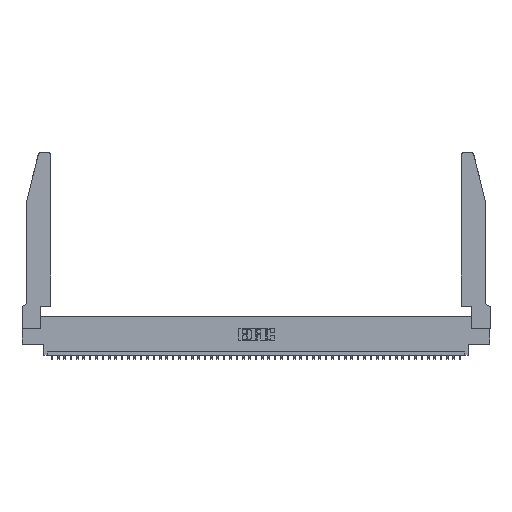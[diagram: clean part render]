
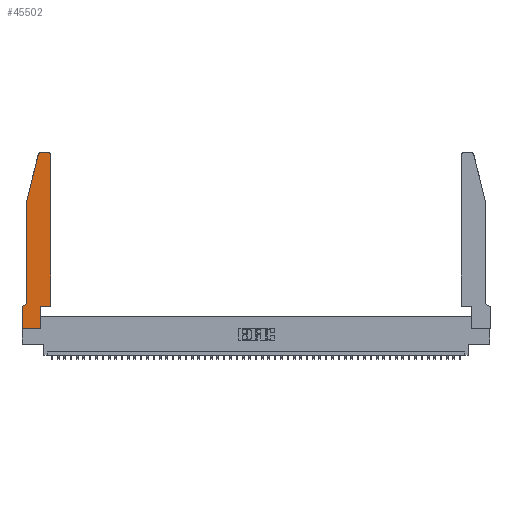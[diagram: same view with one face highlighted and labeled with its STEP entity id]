
A CAD part, top view. The second image highlights one B-rep face of the part: STEP entity #45502.
In plain terms, the highlighted planar face has unit normal (0, 0, 1).
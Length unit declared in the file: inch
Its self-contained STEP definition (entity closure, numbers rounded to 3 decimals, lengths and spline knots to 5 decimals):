
#623 = ORIENTED_EDGE ( 'NONE', *, *, #5632, .T. ) ;
#687 = VECTOR ( 'NONE', #29431, 39.37008 ) ;
#1785 = VECTOR ( 'NONE', #20263, 39.37008 ) ;
#2101 = CARTESIAN_POINT ( 'NONE',  ( 0.0755, 0.35, 0.37 ) ) ;
#2113 = VERTEX_POINT ( 'NONE', #43645 ) ;
#3459 = DIRECTION ( 'NONE',  ( 0., 1., 0. ) ) ;
#4169 = VERTEX_POINT ( 'NONE', #6044 ) ;
#4292 = EDGE_CURVE ( 'NONE', #4169, #29714, #37323, .T. ) ;
#4338 = ORIENTED_EDGE ( 'NONE', *, *, #27550, .T. ) ;
#5632 = EDGE_CURVE ( 'NONE', #13591, #13828, #32533, .T. ) ;
#5811 = VECTOR ( 'NONE', #3459, 39.37008 ) ;
#6044 = CARTESIAN_POINT ( 'NONE',  ( 0.2865, 0.35, 0.37 ) ) ;
#6108 = CARTESIAN_POINT ( 'NONE',  ( 0.4505, 2.72, 0.37 ) ) ;
#6437 = EDGE_CURVE ( 'NONE', #47533, #32549, #17622, .T. ) ;
#6633 = CARTESIAN_POINT ( 'NONE',  ( 0.4205, 2.75, 0.37 ) ) ;
#7588 = CARTESIAN_POINT ( 'NONE',  ( 0.284, 2.75, 0.37 ) ) ;
#7615 = ORIENTED_EDGE ( 'NONE', *, *, #19950, .T. ) ;
#7971 = CIRCLE ( 'NONE', #9192, 0.03 ) ;
#8495 = ORIENTED_EDGE ( 'NONE', *, *, #27144, .T. ) ;
#9192 = AXIS2_PLACEMENT_3D ( 'NONE', #14152, #41817, #18225 ) ;
#10616 = AXIS2_PLACEMENT_3D ( 'NONE', #16713, #36982, #32353 ) ;
#10775 = EDGE_CURVE ( 'NONE', #32549, #2113, #27629, .T. ) ;
#11561 = EDGE_CURVE ( 'NONE', #2113, #14664, #46211, .T. ) ;
#12691 = LINE ( 'NONE', #15873, #40345 ) ;
#13591 = VERTEX_POINT ( 'NONE', #37163 ) ;
#13828 = VERTEX_POINT ( 'NONE', #41092 ) ;
#13968 = VERTEX_POINT ( 'NONE', #6108 ) ;
#14152 = CARTESIAN_POINT ( 'NONE',  ( 0.4205, 2.72, 0.37 ) ) ;
#14617 = CARTESIAN_POINT ( 'NONE',  ( 0.2865, 0., 0.37 ) ) ;
#14664 = VERTEX_POINT ( 'NONE', #48124 ) ;
#14919 = DIRECTION ( 'NONE',  ( -1., 0., 0. ) ) ;
#15873 = CARTESIAN_POINT ( 'NONE',  ( 0., 0., 0.37 ) ) ;
#16177 = LINE ( 'NONE', #49086, #5811 ) ;
#16605 = VECTOR ( 'NONE', #21798, 39.37008 ) ;
#16713 = CARTESIAN_POINT ( 'NONE',  ( 0.284, 2.72, 0.37 ) ) ;
#17416 = CIRCLE ( 'NONE', #38497, 0.07 ) ;
#17622 = LINE ( 'NONE', #23286, #42280 ) ;
#18009 = VECTOR ( 'NONE', #47595, 39.37008 ) ;
#18132 = CARTESIAN_POINT ( 'NONE',  ( 0.0055, 0.42, 0.37 ) ) ;
#18225 = DIRECTION ( 'NONE',  ( 1., 0., 0. ) ) ;
#18475 = AXIS2_PLACEMENT_3D ( 'NONE', #46238, #22620, #26442 ) ;
#18809 = EDGE_CURVE ( 'NONE', #20837, #13591, #17416, .T. ) ;
#19408 = LINE ( 'NONE', #32535, #1785 ) ;
#19950 = EDGE_CURVE ( 'NONE', #22151, #4169, #16177, .T. ) ;
#20263 = DIRECTION ( 'NONE',  ( 0., 1., 0. ) ) ;
#20837 = VERTEX_POINT ( 'NONE', #39372 ) ;
#21798 = DIRECTION ( 'NONE',  ( -0.239, -0.971, 0. ) ) ;
#22138 = CARTESIAN_POINT ( 'NONE',  ( 0., 0., 0.37 ) ) ;
#22151 = VERTEX_POINT ( 'NONE', #14617 ) ;
#22620 = DIRECTION ( 'NONE',  ( 0., 0., 1. ) ) ;
#23242 = ORIENTED_EDGE ( 'NONE', *, *, #10775, .T. ) ;
#23286 = CARTESIAN_POINT ( 'NONE',  ( 0.2605, 2.75, 0.37 ) ) ;
#23690 = ORIENTED_EDGE ( 'NONE', *, *, #18809, .T. ) ;
#24366 = FACE_OUTER_BOUND ( 'NONE', #28994, .T. ) ;
#25699 = DIRECTION ( 'NONE',  ( -1., 0., 0. ) ) ;
#26376 = DIRECTION ( 'NONE',  ( 1., 0., 0. ) ) ;
#26442 = DIRECTION ( 'NONE',  ( 1., 0., 0. ) ) ;
#26876 = VECTOR ( 'NONE', #45361, 39.37008 ) ;
#27144 = EDGE_CURVE ( 'NONE', #13968, #47533, #7971, .T. ) ;
#27550 = EDGE_CURVE ( 'NONE', #14664, #20837, #29940, .T. ) ;
#27629 = CIRCLE ( 'NONE', #10616, 0.03 ) ;
#28217 = ORIENTED_EDGE ( 'NONE', *, *, #46300, .T. ) ;
#28828 = CARTESIAN_POINT ( 'NONE',  ( 0., 0., 0.37 ) ) ;
#28994 = EDGE_LOOP ( 'NONE', ( #43393, #23242, #30224, #4338, #23690, #623, #28217, #44452, #7615, #42724, #46338, #8495 ) ) ;
#29431 = DIRECTION ( 'NONE',  ( -1., 0., 0. ) ) ;
#29534 = DIRECTION ( 'NONE',  ( 0., 0., -1. ) ) ;
#29543 = CARTESIAN_POINT ( 'NONE',  ( 0.0755, 2., 0.37 ) ) ;
#29606 = CARTESIAN_POINT ( 'NONE',  ( 0.0755, 2., 0.37 ) ) ;
#29714 = VERTEX_POINT ( 'NONE', #31442 ) ;
#29940 = LINE ( 'NONE', #29543, #26876 ) ;
#30008 = EDGE_CURVE ( 'NONE', #35655, #22151, #32218, .T. ) ;
#30224 = ORIENTED_EDGE ( 'NONE', *, *, #11561, .T. ) ;
#31442 = CARTESIAN_POINT ( 'NONE',  ( 0.4505, 0.35, 0.37 ) ) ;
#32218 = LINE ( 'NONE', #22138, #18009 ) ;
#32353 = DIRECTION ( 'NONE',  ( 1., 0., 0. ) ) ;
#32533 = LINE ( 'NONE', #2101, #687 ) ;
#32535 = CARTESIAN_POINT ( 'NONE',  ( 0.4505, 0.35, 0.37 ) ) ;
#32549 = VERTEX_POINT ( 'NONE', #7588 ) ;
#34876 = VECTOR ( 'NONE', #26376, 39.37008 ) ;
#35655 = VERTEX_POINT ( 'NONE', #28828 ) ;
#36982 = DIRECTION ( 'NONE',  ( 0., 0., 1. ) ) ;
#37163 = CARTESIAN_POINT ( 'NONE',  ( 0.0055, 0.35, 0.37 ) ) ;
#37323 = LINE ( 'NONE', #49960, #34876 ) ;
#38497 = AXIS2_PLACEMENT_3D ( 'NONE', #18132, #29534, #25699 ) ;
#39372 = CARTESIAN_POINT ( 'NONE',  ( 0.0755, 0.42, 0.37 ) ) ;
#39767 = DIRECTION ( 'NONE',  ( 0., -1., 0. ) ) ;
#40345 = VECTOR ( 'NONE', #39767, 39.37008 ) ;
#41092 = CARTESIAN_POINT ( 'NONE',  ( 0., 0.35, 0.37 ) ) ;
#41817 = DIRECTION ( 'NONE',  ( 0., 0., 1. ) ) ;
#42111 = EDGE_CURVE ( 'NONE', #29714, #13968, #19408, .T. ) ;
#42280 = VECTOR ( 'NONE', #14919, 39.37008 ) ;
#42724 = ORIENTED_EDGE ( 'NONE', *, *, #4292, .T. ) ;
#43393 = ORIENTED_EDGE ( 'NONE', *, *, #6437, .T. ) ;
#43645 = CARTESIAN_POINT ( 'NONE',  ( 0.25487, 2.72718, 0.37 ) ) ;
#44452 = ORIENTED_EDGE ( 'NONE', *, *, #30008, .T. ) ;
#45361 = DIRECTION ( 'NONE',  ( 0., -1., 0. ) ) ;
#45502 = ADVANCED_FACE ( 'NONE', ( #24366 ), #50533, .T. ) ;
#46211 = LINE ( 'NONE', #29606, #16605 ) ;
#46238 = CARTESIAN_POINT ( 'NONE',  ( 0., 0.35, 0.37 ) ) ;
#46300 = EDGE_CURVE ( 'NONE', #13828, #35655, #12691, .T. ) ;
#46338 = ORIENTED_EDGE ( 'NONE', *, *, #42111, .T. ) ;
#47533 = VERTEX_POINT ( 'NONE', #6633 ) ;
#47595 = DIRECTION ( 'NONE',  ( 1., 0., 0. ) ) ;
#48124 = CARTESIAN_POINT ( 'NONE',  ( 0.0755, 2., 0.37 ) ) ;
#49086 = CARTESIAN_POINT ( 'NONE',  ( 0.2865, 0.35, 0.37 ) ) ;
#49960 = CARTESIAN_POINT ( 'NONE',  ( 0.4505, 0.35, 0.37 ) ) ;
#50533 = PLANE ( 'NONE',  #18475 ) ;
